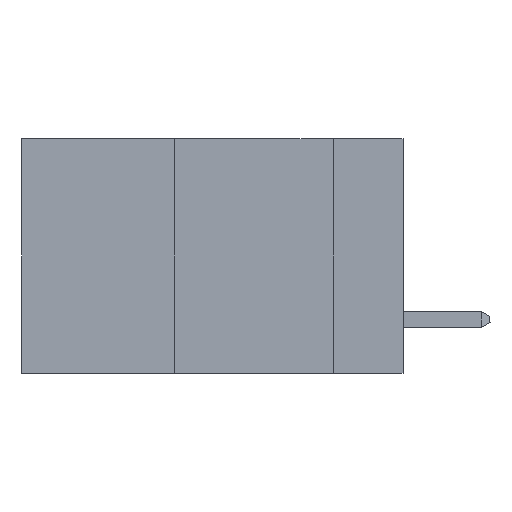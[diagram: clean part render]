
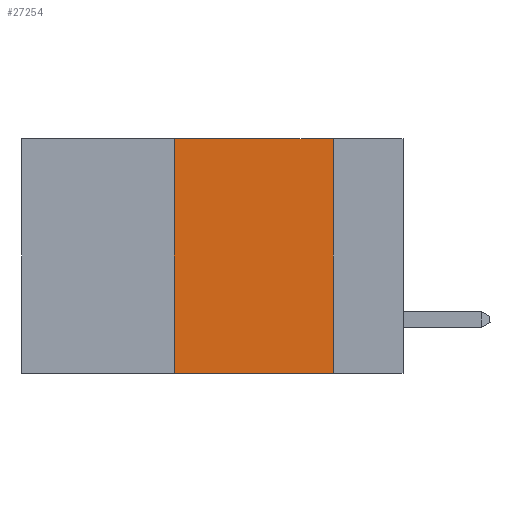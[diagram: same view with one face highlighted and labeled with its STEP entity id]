
A CAD part, left-side view. The second image highlights one B-rep face of the part: STEP entity #27254.
In plain terms, the highlighted planar face has unit normal (-1, 0, 0).
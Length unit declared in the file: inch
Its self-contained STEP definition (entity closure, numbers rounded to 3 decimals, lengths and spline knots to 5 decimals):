
#500 = EDGE_CURVE ( 'NONE', #8594, #2744, #21478, .T. ) ;
#614 = DIRECTION ( 'NONE',  ( 0., 0., 1. ) ) ;
#740 = DIRECTION ( 'NONE',  ( 1., 0., 0. ) ) ;
#982 = CARTESIAN_POINT ( 'NONE',  ( 0., 0.6, -0.37 ) ) ;
#1309 = VECTOR ( 'NONE', #3352, 39.37008 ) ;
#1338 = DIRECTION ( 'NONE',  ( 0., 0., -1. ) ) ;
#2184 = LINE ( 'NONE', #982, #3864 ) ;
#2355 = FACE_OUTER_BOUND ( 'NONE', #16837, .T. ) ;
#2744 = VERTEX_POINT ( 'NONE', #18430 ) ;
#2939 = VERTEX_POINT ( 'NONE', #15290 ) ;
#3352 = DIRECTION ( 'NONE',  ( 0., -1., 0. ) ) ;
#3864 = VECTOR ( 'NONE', #5186, 39.37008 ) ;
#3940 = ORIENTED_EDGE ( 'NONE', *, *, #8814, .F. ) ;
#5186 = DIRECTION ( 'NONE',  ( 0., -1., 0. ) ) ;
#5189 = CARTESIAN_POINT ( 'NONE',  ( 0., 0.11, -0.37 ) ) ;
#5281 = VERTEX_POINT ( 'NONE', #5189 ) ;
#7288 = CARTESIAN_POINT ( 'NONE',  ( 0., 0.6, 0. ) ) ;
#7550 = ORIENTED_EDGE ( 'NONE', *, *, #500, .F. ) ;
#8594 = VERTEX_POINT ( 'NONE', #24009 ) ;
#8814 = EDGE_CURVE ( 'NONE', #2744, #2939, #27137, .T. ) ;
#12827 = ORIENTED_EDGE ( 'NONE', *, *, #21577, .T. ) ;
#13148 = ORIENTED_EDGE ( 'NONE', *, *, #27286, .F. ) ;
#14295 = LINE ( 'NONE', #17984, #24899 ) ;
#15233 = AXIS2_PLACEMENT_3D ( 'NONE', #7288, #740, #24039 ) ;
#15290 = CARTESIAN_POINT ( 'NONE',  ( 0., 0.11, 0. ) ) ;
#16837 = EDGE_LOOP ( 'NONE', ( #13148, #3940, #7550, #12827 ) ) ;
#17459 = CARTESIAN_POINT ( 'NONE',  ( 0., 0.36, 0. ) ) ;
#17984 = CARTESIAN_POINT ( 'NONE',  ( 0., 0.11, 0. ) ) ;
#18430 = CARTESIAN_POINT ( 'NONE',  ( 0., 0.36, 0. ) ) ;
#19470 = VECTOR ( 'NONE', #614, 39.37008 ) ;
#19732 = CARTESIAN_POINT ( 'NONE',  ( 0., 0.6, 0. ) ) ;
#21478 = LINE ( 'NONE', #17459, #19470 ) ;
#21577 = EDGE_CURVE ( 'NONE', #8594, #5281, #2184, .T. ) ;
#24009 = CARTESIAN_POINT ( 'NONE',  ( 0., 0.36, -0.37 ) ) ;
#24039 = DIRECTION ( 'NONE',  ( 0., 0., -1. ) ) ;
#24899 = VECTOR ( 'NONE', #1338, 39.37008 ) ;
#26254 = PLANE ( 'NONE',  #15233 ) ;
#27137 = LINE ( 'NONE', #19732, #1309 ) ;
#27254 = ADVANCED_FACE ( 'NONE', ( #2355 ), #26254, .F. ) ;
#27286 = EDGE_CURVE ( 'NONE', #2939, #5281, #14295, .T. ) ;
